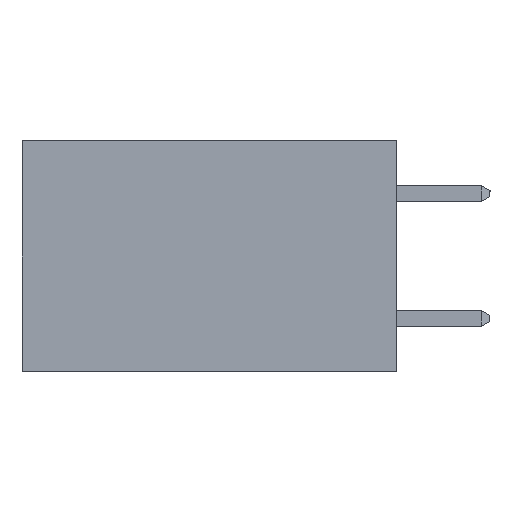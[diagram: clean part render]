
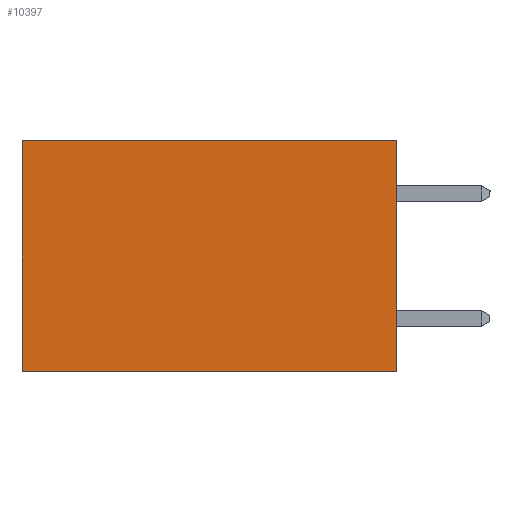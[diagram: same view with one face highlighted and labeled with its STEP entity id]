
A CAD part, left-side view. The second image highlights one B-rep face of the part: STEP entity #10397.
In plain terms, the highlighted planar face has unit normal (-1, 0, 0).
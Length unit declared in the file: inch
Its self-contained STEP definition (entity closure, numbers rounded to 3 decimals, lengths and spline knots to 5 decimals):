
#932 = VERTEX_POINT ( 'NONE', #4615 ) ;
#1753 = CARTESIAN_POINT ( 'NONE',  ( 0.2615, 0., -0.37 ) ) ;
#2083 = VERTEX_POINT ( 'NONE', #12890 ) ;
#2115 = DIRECTION ( 'NONE',  ( 0., 1., 0. ) ) ;
#4309 = ORIENTED_EDGE ( 'NONE', *, *, #4342, .T. ) ;
#4342 = EDGE_CURVE ( 'NONE', #16430, #9520, #20895, .T. ) ;
#4615 = CARTESIAN_POINT ( 'NONE',  ( 0.2615, 0.6, -0.37 ) ) ;
#5062 = ORIENTED_EDGE ( 'NONE', *, *, #13592, .T. ) ;
#5077 = DIRECTION ( 'NONE',  ( 0., 0., -1. ) ) ;
#5727 = VECTOR ( 'NONE', #16998, 39.37008 ) ;
#6302 = CARTESIAN_POINT ( 'NONE',  ( 0.2615, 0., -0.37 ) ) ;
#7233 = EDGE_CURVE ( 'NONE', #16430, #2083, #10339, .T. ) ;
#8696 = CARTESIAN_POINT ( 'NONE',  ( 0.2615, 0., 0. ) ) ;
#9183 = DIRECTION ( 'NONE',  ( 0., 0., -1. ) ) ;
#9520 = VERTEX_POINT ( 'NONE', #21854 ) ;
#9567 = FACE_OUTER_BOUND ( 'NONE', #11877, .T. ) ;
#9693 = DIRECTION ( 'NONE',  ( 1., 0., 0. ) ) ;
#10339 = LINE ( 'NONE', #6302, #16150 ) ;
#10397 = ADVANCED_FACE ( 'NONE', ( #9567 ), #19597, .F. ) ;
#10996 = CARTESIAN_POINT ( 'NONE',  ( 0.2615, 0., 0. ) ) ;
#11877 = EDGE_LOOP ( 'NONE', ( #5062, #20436, #18888, #4309 ) ) ;
#12890 = CARTESIAN_POINT ( 'NONE',  ( 0.2615, 0., -0.37 ) ) ;
#13271 = LINE ( 'NONE', #14715, #24214 ) ;
#13592 = EDGE_CURVE ( 'NONE', #9520, #932, #13271, .T. ) ;
#13961 = LINE ( 'NONE', #19963, #24053 ) ;
#14715 = CARTESIAN_POINT ( 'NONE',  ( 0.2615, 0.6, -0.37 ) ) ;
#16150 = VECTOR ( 'NONE', #16189, 39.37008 ) ;
#16189 = DIRECTION ( 'NONE',  ( 0., 0., -1. ) ) ;
#16430 = VERTEX_POINT ( 'NONE', #8696 ) ;
#16998 = DIRECTION ( 'NONE',  ( 0., 1., 0. ) ) ;
#18340 = AXIS2_PLACEMENT_3D ( 'NONE', #1753, #9693, #9183 ) ;
#18888 = ORIENTED_EDGE ( 'NONE', *, *, #7233, .F. ) ;
#19597 = PLANE ( 'NONE',  #18340 ) ;
#19963 = CARTESIAN_POINT ( 'NONE',  ( 0.2615, 0., -0.37 ) ) ;
#20436 = ORIENTED_EDGE ( 'NONE', *, *, #23003, .F. ) ;
#20895 = LINE ( 'NONE', #10996, #5727 ) ;
#21854 = CARTESIAN_POINT ( 'NONE',  ( 0.2615, 0.6, 0. ) ) ;
#23003 = EDGE_CURVE ( 'NONE', #2083, #932, #13961, .T. ) ;
#24053 = VECTOR ( 'NONE', #2115, 39.37008 ) ;
#24214 = VECTOR ( 'NONE', #5077, 39.37008 ) ;
